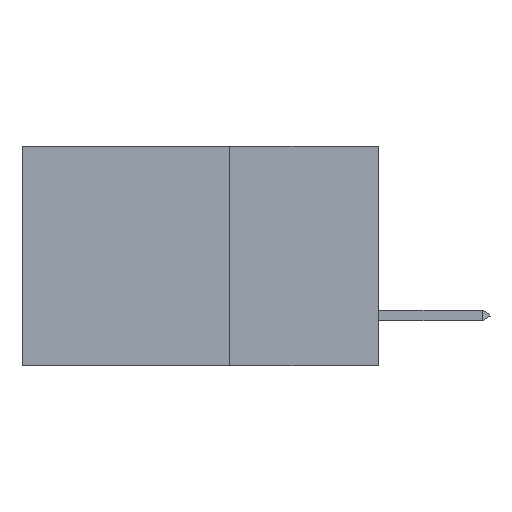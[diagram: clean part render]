
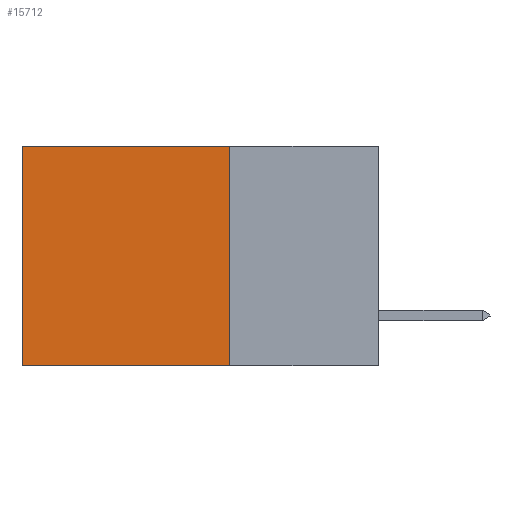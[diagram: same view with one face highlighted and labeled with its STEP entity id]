
A CAD part, left-side view. The second image highlights one B-rep face of the part: STEP entity #15712.
In plain terms, the highlighted planar face has unit normal (-1, 0, 0).
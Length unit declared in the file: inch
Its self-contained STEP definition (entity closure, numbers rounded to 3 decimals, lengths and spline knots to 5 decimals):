
#346 = ORIENTED_EDGE ( 'NONE', *, *, #10984, .F. ) ;
#621 = VECTOR ( 'NONE', #2745, 39.37008 ) ;
#1854 = VECTOR ( 'NONE', #8805, 39.37008 ) ;
#2696 = CARTESIAN_POINT ( 'NONE',  ( 0.298, 0.25, -0.37 ) ) ;
#2745 = DIRECTION ( 'NONE',  ( 0., 1., 0. ) ) ;
#2849 = LINE ( 'NONE', #2696, #17537 ) ;
#2859 = ORIENTED_EDGE ( 'NONE', *, *, #13099, .T. ) ;
#2959 = ORIENTED_EDGE ( 'NONE', *, *, #5616, .F. ) ;
#4338 = CARTESIAN_POINT ( 'NONE',  ( 0.298, 0.25, 0. ) ) ;
#4568 = ORIENTED_EDGE ( 'NONE', *, *, #8492, .T. ) ;
#5616 = EDGE_CURVE ( 'NONE', #6063, #9693, #17969, .T. ) ;
#5652 = DIRECTION ( 'NONE',  ( 0., 1., 0. ) ) ;
#5919 = CARTESIAN_POINT ( 'NONE',  ( 0.298, 0.25, 0. ) ) ;
#6063 = VERTEX_POINT ( 'NONE', #5919 ) ;
#6260 = VECTOR ( 'NONE', #11595, 39.37008 ) ;
#7043 = CARTESIAN_POINT ( 'NONE',  ( 0.298, 0.25, 0. ) ) ;
#7503 = CARTESIAN_POINT ( 'NONE',  ( 0.298, 0.6, 0. ) ) ;
#8285 = LINE ( 'NONE', #7503, #1854 ) ;
#8492 = EDGE_CURVE ( 'NONE', #6063, #12983, #10716, .T. ) ;
#8789 = CARTESIAN_POINT ( 'NONE',  ( 0.298, 0.25, -0.37 ) ) ;
#8805 = DIRECTION ( 'NONE',  ( 0., 0., -1. ) ) ;
#9074 = PLANE ( 'NONE',  #11411 ) ;
#9693 = VERTEX_POINT ( 'NONE', #8789 ) ;
#10716 = LINE ( 'NONE', #4338, #621 ) ;
#10984 = EDGE_CURVE ( 'NONE', #9693, #13946, #2849, .T. ) ;
#11411 = AXIS2_PLACEMENT_3D ( 'NONE', #11845, #14649, #17679 ) ;
#11595 = DIRECTION ( 'NONE',  ( 0., 0., -1. ) ) ;
#11833 = FACE_OUTER_BOUND ( 'NONE', #16406, .T. ) ;
#11845 = CARTESIAN_POINT ( 'NONE',  ( 0.298, 0.25, 0. ) ) ;
#12983 = VERTEX_POINT ( 'NONE', #15503 ) ;
#13099 = EDGE_CURVE ( 'NONE', #12983, #13946, #8285, .T. ) ;
#13946 = VERTEX_POINT ( 'NONE', #18781 ) ;
#14649 = DIRECTION ( 'NONE',  ( 1., 0., 0. ) ) ;
#15503 = CARTESIAN_POINT ( 'NONE',  ( 0.298, 0.6, 0. ) ) ;
#15712 = ADVANCED_FACE ( 'NONE', ( #11833 ), #9074, .F. ) ;
#16406 = EDGE_LOOP ( 'NONE', ( #2859, #346, #2959, #4568 ) ) ;
#17537 = VECTOR ( 'NONE', #5652, 39.37008 ) ;
#17679 = DIRECTION ( 'NONE',  ( 0., 0., -1. ) ) ;
#17969 = LINE ( 'NONE', #7043, #6260 ) ;
#18781 = CARTESIAN_POINT ( 'NONE',  ( 0.298, 0.6, -0.37 ) ) ;
